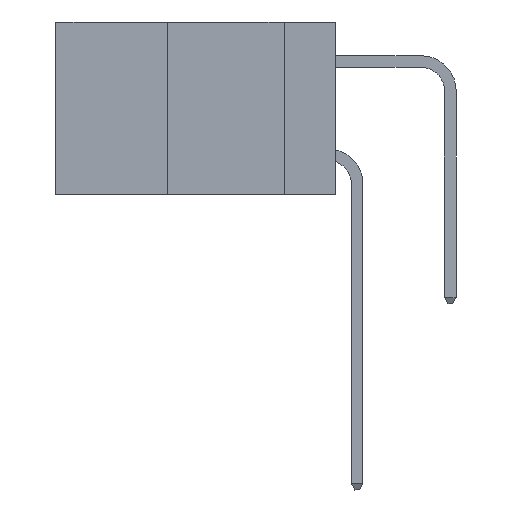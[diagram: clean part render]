
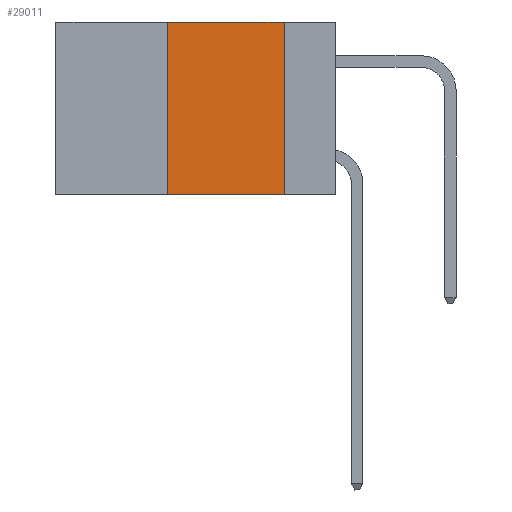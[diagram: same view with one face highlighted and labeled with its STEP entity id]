
A CAD part, left-side view. The second image highlights one B-rep face of the part: STEP entity #29011.
In plain terms, the highlighted planar face has unit normal (-1, 0, 0).
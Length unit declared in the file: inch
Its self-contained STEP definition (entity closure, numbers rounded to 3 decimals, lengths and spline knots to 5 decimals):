
#1026 = EDGE_CURVE ( 'NONE', #32342, #3189, #24746, .T. ) ;
#1779 = EDGE_CURVE ( 'NONE', #32342, #3717, #7829, .T. ) ;
#2346 = DIRECTION ( 'NONE',  ( 1., 0., 0. ) ) ;
#3189 = VERTEX_POINT ( 'NONE', #26134 ) ;
#3717 = VERTEX_POINT ( 'NONE', #13072 ) ;
#6966 = ORIENTED_EDGE ( 'NONE', *, *, #26322, .F. ) ;
#7829 = LINE ( 'NONE', #24689, #30399 ) ;
#7896 = DIRECTION ( 'NONE',  ( 0., -1., 0. ) ) ;
#8729 = VECTOR ( 'NONE', #25452, 39.37008 ) ;
#9179 = ORIENTED_EDGE ( 'NONE', *, *, #1026, .F. ) ;
#9562 = VERTEX_POINT ( 'NONE', #13924 ) ;
#9799 = CARTESIAN_POINT ( 'NONE',  ( 0., 0.36, 0. ) ) ;
#11815 = DIRECTION ( 'NONE',  ( 0., -1., 0. ) ) ;
#12570 = FACE_OUTER_BOUND ( 'NONE', #26464, .T. ) ;
#12573 = CARTESIAN_POINT ( 'NONE',  ( 0., 0.11, 0. ) ) ;
#12682 = CARTESIAN_POINT ( 'NONE',  ( 0., 0.36, -0.37 ) ) ;
#13070 = VECTOR ( 'NONE', #32687, 39.37008 ) ;
#13072 = CARTESIAN_POINT ( 'NONE',  ( 0., 0.11, -0.37 ) ) ;
#13924 = CARTESIAN_POINT ( 'NONE',  ( 0., 0.11, 0. ) ) ;
#14720 = LINE ( 'NONE', #28211, #22424 ) ;
#14838 = ORIENTED_EDGE ( 'NONE', *, *, #1779, .T. ) ;
#17939 = DIRECTION ( 'NONE',  ( 0., 0., -1. ) ) ;
#17994 = EDGE_CURVE ( 'NONE', #9562, #3717, #22498, .T. ) ;
#19602 = AXIS2_PLACEMENT_3D ( 'NONE', #25956, #2346, #17939 ) ;
#22424 = VECTOR ( 'NONE', #7896, 39.37008 ) ;
#22498 = LINE ( 'NONE', #12573, #8729 ) ;
#24689 = CARTESIAN_POINT ( 'NONE',  ( 0., 0.6, -0.37 ) ) ;
#24746 = LINE ( 'NONE', #9799, #13070 ) ;
#25452 = DIRECTION ( 'NONE',  ( 0., 0., -1. ) ) ;
#25956 = CARTESIAN_POINT ( 'NONE',  ( 0., 0.6, 0. ) ) ;
#26134 = CARTESIAN_POINT ( 'NONE',  ( 0., 0.36, 0. ) ) ;
#26322 = EDGE_CURVE ( 'NONE', #3189, #9562, #14720, .T. ) ;
#26464 = EDGE_LOOP ( 'NONE', ( #29449, #6966, #9179, #14838 ) ) ;
#28211 = CARTESIAN_POINT ( 'NONE',  ( 0., 0.6, 0. ) ) ;
#29011 = ADVANCED_FACE ( 'NONE', ( #12570 ), #30935, .F. ) ;
#29449 = ORIENTED_EDGE ( 'NONE', *, *, #17994, .F. ) ;
#30399 = VECTOR ( 'NONE', #11815, 39.37008 ) ;
#30935 = PLANE ( 'NONE',  #19602 ) ;
#32342 = VERTEX_POINT ( 'NONE', #12682 ) ;
#32687 = DIRECTION ( 'NONE',  ( 0., 0., 1. ) ) ;
